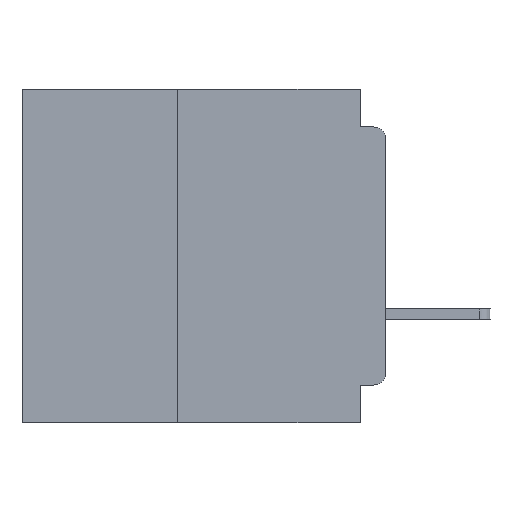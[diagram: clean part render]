
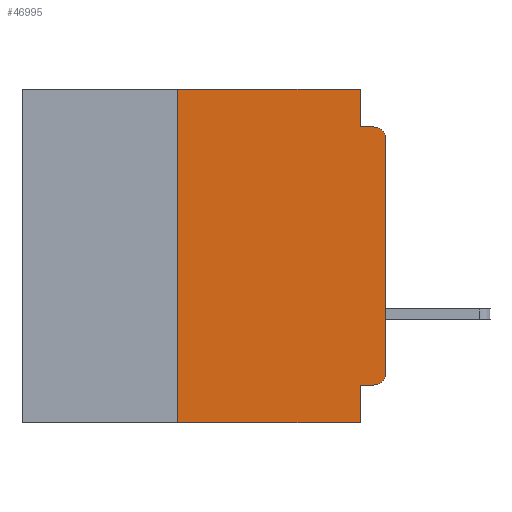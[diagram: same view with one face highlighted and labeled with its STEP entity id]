
A CAD part, left-side view. The second image highlights one B-rep face of the part: STEP entity #46995.
In plain terms, the highlighted planar face has unit normal (-1, 0, 0).
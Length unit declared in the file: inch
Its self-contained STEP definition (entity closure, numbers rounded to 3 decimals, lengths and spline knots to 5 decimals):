
#548 = VECTOR ( 'NONE', #68216, 39.37008 ) ;
#2861 = VERTEX_POINT ( 'NONE', #42532 ) ;
#5321 = ORIENTED_EDGE ( 'NONE', *, *, #7284, .F. ) ;
#5480 = CARTESIAN_POINT ( 'NONE',  ( 0., 0.031, -0.4 ) ) ;
#6125 = ORIENTED_EDGE ( 'NONE', *, *, #9117, .F. ) ;
#7284 = EDGE_CURVE ( 'NONE', #29595, #61493, #17765, .T. ) ;
#9094 = VERTEX_POINT ( 'NONE', #40125 ) ;
#9117 = EDGE_CURVE ( 'NONE', #61793, #59236, #39853, .T. ) ;
#9139 = CARTESIAN_POINT ( 'NONE',  ( 0., 0.015, -0.06 ) ) ;
#9422 = CARTESIAN_POINT ( 'NONE',  ( 0., 0.25, -0.4 ) ) ;
#10472 = VERTEX_POINT ( 'NONE', #29687 ) ;
#11158 = CARTESIAN_POINT ( 'NONE',  ( 0., 0.015, -0.355 ) ) ;
#11825 = ORIENTED_EDGE ( 'NONE', *, *, #15272, .F. ) ;
#13301 = CARTESIAN_POINT ( 'NONE',  ( 0., 0.25, 0. ) ) ;
#13307 = CARTESIAN_POINT ( 'NONE',  ( 0., 0.437, 0. ) ) ;
#13539 = CARTESIAN_POINT ( 'NONE',  ( 0., 0.031, 0. ) ) ;
#14480 = DIRECTION ( 'NONE',  ( 0., 0., -1. ) ) ;
#15272 = EDGE_CURVE ( 'NONE', #10472, #9094, #32639, .T. ) ;
#15340 = VECTOR ( 'NONE', #25381, 39.37008 ) ;
#17765 = LINE ( 'NONE', #9422, #58182 ) ;
#22938 = CARTESIAN_POINT ( 'NONE',  ( 0., 0.437, 0. ) ) ;
#24761 = ORIENTED_EDGE ( 'NONE', *, *, #35642, .F. ) ;
#25381 = DIRECTION ( 'NONE',  ( 0., -1., 0. ) ) ;
#26264 = LINE ( 'NONE', #47328, #66640 ) ;
#26437 = ORIENTED_EDGE ( 'NONE', *, *, #33527, .T. ) ;
#28219 = DIRECTION ( 'NONE',  ( 0., -1., 0. ) ) ;
#28549 = LINE ( 'NONE', #62953, #548 ) ;
#28691 = DIRECTION ( 'NONE',  ( -1., 0., 0. ) ) ;
#29155 = PLANE ( 'NONE',  #34925 ) ;
#29595 = VERTEX_POINT ( 'NONE', #61279 ) ;
#29687 = CARTESIAN_POINT ( 'NONE',  ( 0., 0.031, -0.045 ) ) ;
#30180 = EDGE_CURVE ( 'NONE', #61793, #66883, #58019, .T. ) ;
#31463 = ORIENTED_EDGE ( 'NONE', *, *, #56304, .F. ) ;
#32639 = LINE ( 'NONE', #51711, #15340 ) ;
#32711 = VERTEX_POINT ( 'NONE', #13539 ) ;
#33527 = EDGE_CURVE ( 'NONE', #29595, #48407, #26264, .T. ) ;
#33894 = FACE_OUTER_BOUND ( 'NONE', #66088, .T. ) ;
#34321 = VECTOR ( 'NONE', #48109, 39.37008 ) ;
#34439 = ORIENTED_EDGE ( 'NONE', *, *, #66201, .T. ) ;
#34465 = DIRECTION ( 'NONE',  ( 0., 0., -1. ) ) ;
#34925 = AXIS2_PLACEMENT_3D ( 'NONE', #13307, #66023, #34465 ) ;
#35642 = EDGE_CURVE ( 'NONE', #61493, #32711, #67715, .T. ) ;
#36495 = DIRECTION ( 'NONE',  ( 0., 0., -1. ) ) ;
#37191 = AXIS2_PLACEMENT_3D ( 'NONE', #60299, #28691, #65539 ) ;
#38817 = ORIENTED_EDGE ( 'NONE', *, *, #42428, .F. ) ;
#39729 = VECTOR ( 'NONE', #28219, 39.37008 ) ;
#39853 = LINE ( 'NONE', #56274, #52287 ) ;
#40125 = CARTESIAN_POINT ( 'NONE',  ( 0., 0.015, -0.045 ) ) ;
#41689 = CARTESIAN_POINT ( 'NONE',  ( 0., 0., -0.34 ) ) ;
#42428 = EDGE_CURVE ( 'NONE', #32711, #10472, #63984, .T. ) ;
#42532 = CARTESIAN_POINT ( 'NONE',  ( 0., 0., -0.06 ) ) ;
#42783 = CARTESIAN_POINT ( 'NONE',  ( 0., 0.031, 0. ) ) ;
#43856 = AXIS2_PLACEMENT_3D ( 'NONE', #9139, #46089, #14480 ) ;
#44739 = LINE ( 'NONE', #62791, #57097 ) ;
#44787 = CIRCLE ( 'NONE', #43856, 0.015 ) ;
#46089 = DIRECTION ( 'NONE',  ( -1., 0., 0. ) ) ;
#46383 = DIRECTION ( 'NONE',  ( 0., 0., 1. ) ) ;
#46995 = ADVANCED_FACE ( 'NONE', ( #33894 ), #29155, .F. ) ;
#47328 = CARTESIAN_POINT ( 'NONE',  ( 0., 0.437, -0.4 ) ) ;
#47487 = CARTESIAN_POINT ( 'NONE',  ( 0., 0.031, -0.355 ) ) ;
#48109 = DIRECTION ( 'NONE',  ( 0., 0., -1. ) ) ;
#48407 = VERTEX_POINT ( 'NONE', #5480 ) ;
#51229 = DIRECTION ( 'NONE',  ( 0., 1., 0. ) ) ;
#51711 = CARTESIAN_POINT ( 'NONE',  ( 0., 0., -0.045 ) ) ;
#52287 = VECTOR ( 'NONE', #51229, 39.37008 ) ;
#53368 = ORIENTED_EDGE ( 'NONE', *, *, #58100, .T. ) ;
#56274 = CARTESIAN_POINT ( 'NONE',  ( 0., 0., -0.355 ) ) ;
#56304 = EDGE_CURVE ( 'NONE', #59236, #48407, #44739, .T. ) ;
#57097 = VECTOR ( 'NONE', #36495, 39.37008 ) ;
#58019 = CIRCLE ( 'NONE', #37191, 0.015 ) ;
#58100 = EDGE_CURVE ( 'NONE', #2861, #9094, #44787, .T. ) ;
#58182 = VECTOR ( 'NONE', #46383, 39.37008 ) ;
#59236 = VERTEX_POINT ( 'NONE', #47487 ) ;
#60299 = CARTESIAN_POINT ( 'NONE',  ( 0., 0.015, -0.34 ) ) ;
#61279 = CARTESIAN_POINT ( 'NONE',  ( 0., 0.25, -0.4 ) ) ;
#61437 = ORIENTED_EDGE ( 'NONE', *, *, #30180, .T. ) ;
#61493 = VERTEX_POINT ( 'NONE', #13301 ) ;
#61793 = VERTEX_POINT ( 'NONE', #11158 ) ;
#62791 = CARTESIAN_POINT ( 'NONE',  ( 0., 0.031, -0.4 ) ) ;
#62953 = CARTESIAN_POINT ( 'NONE',  ( 0., 0., 0. ) ) ;
#63984 = LINE ( 'NONE', #42783, #34321 ) ;
#65539 = DIRECTION ( 'NONE',  ( 0., 0., -1. ) ) ;
#66023 = DIRECTION ( 'NONE',  ( 1., 0., 0. ) ) ;
#66088 = EDGE_LOOP ( 'NONE', ( #34439, #53368, #11825, #38817, #24761, #5321, #26437, #31463, #6125, #61437 ) ) ;
#66201 = EDGE_CURVE ( 'NONE', #66883, #2861, #28549, .T. ) ;
#66640 = VECTOR ( 'NONE', #68194, 39.37008 ) ;
#66883 = VERTEX_POINT ( 'NONE', #41689 ) ;
#67715 = LINE ( 'NONE', #22938, #39729 ) ;
#68194 = DIRECTION ( 'NONE',  ( 0., -1., 0. ) ) ;
#68216 = DIRECTION ( 'NONE',  ( 0., 0., 1. ) ) ;
